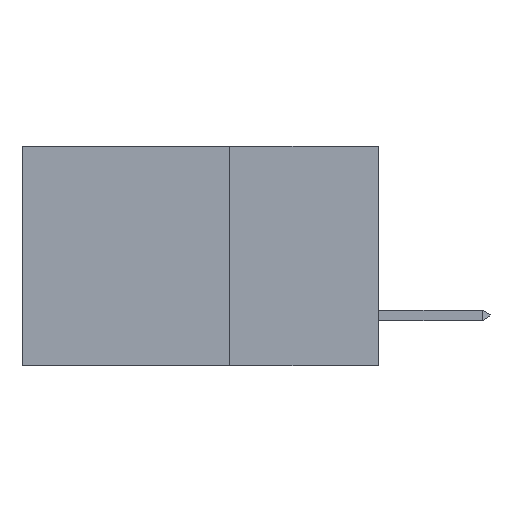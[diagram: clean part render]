
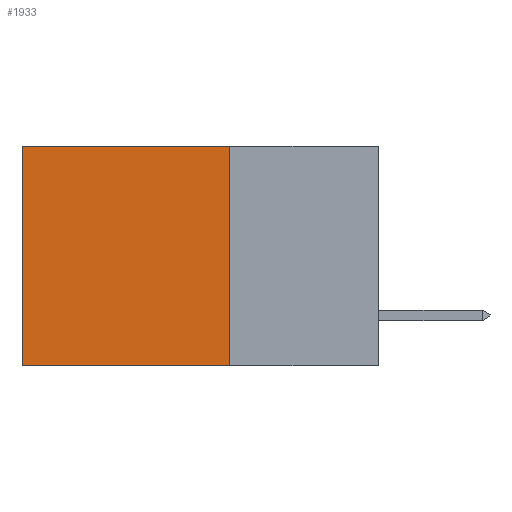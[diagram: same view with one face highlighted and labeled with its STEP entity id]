
A CAD part, left-side view. The second image highlights one B-rep face of the part: STEP entity #1933.
In plain terms, the highlighted planar face has unit normal (-1, 0, 0).
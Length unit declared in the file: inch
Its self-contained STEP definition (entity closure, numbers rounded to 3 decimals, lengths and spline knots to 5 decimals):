
#214 = CARTESIAN_POINT ( 'NONE',  ( 0.2615, 0.25, -0.37 ) ) ;
#1865 = DIRECTION ( 'NONE',  ( 0., 0., -1. ) ) ;
#1933 = ADVANCED_FACE ( 'NONE', ( #23777 ), #23538, .F. ) ;
#2863 = EDGE_LOOP ( 'NONE', ( #19925, #14564, #20752, #23984 ) ) ;
#2936 = VECTOR ( 'NONE', #1865, 39.37008 ) ;
#3374 = CARTESIAN_POINT ( 'NONE',  ( 0.2615, 0.6, 0. ) ) ;
#4527 = DIRECTION ( 'NONE',  ( 0., 1., 0. ) ) ;
#4596 = DIRECTION ( 'NONE',  ( 1., 0., 0. ) ) ;
#4902 = LINE ( 'NONE', #22070, #24003 ) ;
#6122 = CARTESIAN_POINT ( 'NONE',  ( 0.2615, 0.25, -0.37 ) ) ;
#7489 = VERTEX_POINT ( 'NONE', #11162 ) ;
#9527 = EDGE_CURVE ( 'NONE', #17485, #18113, #4902, .T. ) ;
#9762 = CARTESIAN_POINT ( 'NONE',  ( 0.2615, 0.25, -0.37 ) ) ;
#9846 = LINE ( 'NONE', #214, #2936 ) ;
#9884 = EDGE_CURVE ( 'NONE', #17485, #20179, #9846, .T. ) ;
#9900 = CARTESIAN_POINT ( 'NONE',  ( 0.2615, 0.25, 0. ) ) ;
#11162 = CARTESIAN_POINT ( 'NONE',  ( 0.2615, 0.6, -0.37 ) ) ;
#11978 = DIRECTION ( 'NONE',  ( 0., 0., -1. ) ) ;
#13196 = LINE ( 'NONE', #9762, #13250 ) ;
#13250 = VECTOR ( 'NONE', #17380, 39.37008 ) ;
#13327 = EDGE_CURVE ( 'NONE', #18113, #7489, #16411, .T. ) ;
#14564 = ORIENTED_EDGE ( 'NONE', *, *, #22663, .F. ) ;
#15138 = VECTOR ( 'NONE', #22022, 39.37008 ) ;
#16411 = LINE ( 'NONE', #19978, #15138 ) ;
#16569 = AXIS2_PLACEMENT_3D ( 'NONE', #6122, #4596, #11978 ) ;
#17380 = DIRECTION ( 'NONE',  ( 0., 1., 0. ) ) ;
#17485 = VERTEX_POINT ( 'NONE', #9900 ) ;
#18113 = VERTEX_POINT ( 'NONE', #3374 ) ;
#19005 = CARTESIAN_POINT ( 'NONE',  ( 0.2615, 0.25, -0.37 ) ) ;
#19925 = ORIENTED_EDGE ( 'NONE', *, *, #13327, .T. ) ;
#19978 = CARTESIAN_POINT ( 'NONE',  ( 0.2615, 0.6, -0.37 ) ) ;
#20179 = VERTEX_POINT ( 'NONE', #19005 ) ;
#20752 = ORIENTED_EDGE ( 'NONE', *, *, #9884, .F. ) ;
#22022 = DIRECTION ( 'NONE',  ( 0., 0., -1. ) ) ;
#22070 = CARTESIAN_POINT ( 'NONE',  ( 0.2615, 0.25, 0. ) ) ;
#22663 = EDGE_CURVE ( 'NONE', #20179, #7489, #13196, .T. ) ;
#23538 = PLANE ( 'NONE',  #16569 ) ;
#23777 = FACE_OUTER_BOUND ( 'NONE', #2863, .T. ) ;
#23984 = ORIENTED_EDGE ( 'NONE', *, *, #9527, .T. ) ;
#24003 = VECTOR ( 'NONE', #4527, 39.37008 ) ;
